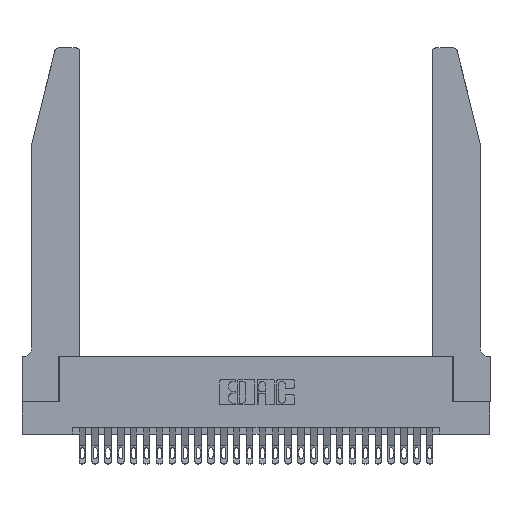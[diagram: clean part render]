
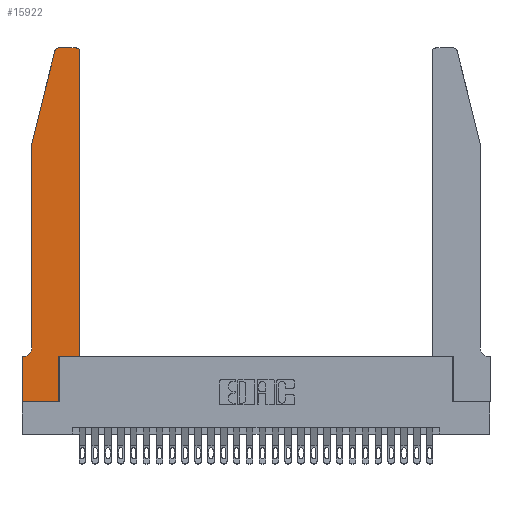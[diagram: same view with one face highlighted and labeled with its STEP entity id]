
A CAD part, top view. The second image highlights one B-rep face of the part: STEP entity #15922.
In plain terms, the highlighted planar face has unit normal (0, 0, 1).
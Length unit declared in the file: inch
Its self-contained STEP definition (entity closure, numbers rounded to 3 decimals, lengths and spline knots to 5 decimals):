
#129 = CARTESIAN_POINT ( 'NONE',  ( 0.2865, 0., 0.37 ) ) ;
#249 = CARTESIAN_POINT ( 'NONE',  ( 0.0755, 2., 0.37 ) ) ;
#687 = VERTEX_POINT ( 'NONE', #129 ) ;
#1228 = EDGE_LOOP ( 'NONE', ( #21166, #9160, #25264, #1572, #23077, #16402, #26009, #11171, #11777, #18417, #9724, #4285 ) ) ;
#1283 = AXIS2_PLACEMENT_3D ( 'NONE', #27763, #12015, #27660 ) ;
#1368 = AXIS2_PLACEMENT_3D ( 'NONE', #26612, #2082, #17727 ) ;
#1412 = DIRECTION ( 'NONE',  ( 1., 0., 0. ) ) ;
#1572 = ORIENTED_EDGE ( 'NONE', *, *, #11192, .T. ) ;
#2082 = DIRECTION ( 'NONE',  ( 0., 0., 1. ) ) ;
#2402 = CARTESIAN_POINT ( 'NONE',  ( 0.4205, 2.75, 0.37 ) ) ;
#2415 = DIRECTION ( 'NONE',  ( 0., -1., 0. ) ) ;
#2513 = AXIS2_PLACEMENT_3D ( 'NONE', #2610, #27211, #5008 ) ;
#2610 = CARTESIAN_POINT ( 'NONE',  ( 0.0055, 0.42, 0.37 ) ) ;
#2716 = LINE ( 'NONE', #18474, #7898 ) ;
#3113 = CARTESIAN_POINT ( 'NONE',  ( 0.2865, 0.35, 0.37 ) ) ;
#3643 = LINE ( 'NONE', #7606, #10619 ) ;
#3847 = VECTOR ( 'NONE', #25803, 39.37008 ) ;
#4285 = ORIENTED_EDGE ( 'NONE', *, *, #13616, .T. ) ;
#4448 = VECTOR ( 'NONE', #22983, 39.37008 ) ;
#4449 = CIRCLE ( 'NONE', #9726, 0.03 ) ;
#4637 = CARTESIAN_POINT ( 'NONE',  ( 0., 0., 0.37 ) ) ;
#5008 = DIRECTION ( 'NONE',  ( -1., 0., 0. ) ) ;
#5041 = CARTESIAN_POINT ( 'NONE',  ( 0.25487, 2.72718, 0.37 ) ) ;
#5281 = EDGE_CURVE ( 'NONE', #6188, #12179, #11892, .T. ) ;
#5611 = CIRCLE ( 'NONE', #1283, 0.03 ) ;
#5969 = CARTESIAN_POINT ( 'NONE',  ( 0., 0., 0.37 ) ) ;
#6003 = CARTESIAN_POINT ( 'NONE',  ( 0.4505, 2.72, 0.37 ) ) ;
#6188 = VERTEX_POINT ( 'NONE', #9576 ) ;
#6628 = VERTEX_POINT ( 'NONE', #5041 ) ;
#6860 = LINE ( 'NONE', #23150, #23339 ) ;
#6877 = EDGE_CURVE ( 'NONE', #20033, #6188, #6860, .T. ) ;
#7310 = CARTESIAN_POINT ( 'NONE',  ( 0.284, 2.75, 0.37 ) ) ;
#7357 = VECTOR ( 'NONE', #15889, 39.37008 ) ;
#7606 = CARTESIAN_POINT ( 'NONE',  ( 0.2605, 2.75, 0.37 ) ) ;
#7898 = VECTOR ( 'NONE', #9640, 39.37008 ) ;
#9097 = VERTEX_POINT ( 'NONE', #7310 ) ;
#9160 = ORIENTED_EDGE ( 'NONE', *, *, #10809, .T. ) ;
#9531 = CARTESIAN_POINT ( 'NONE',  ( 0.4505, 0.35, 0.37 ) ) ;
#9576 = CARTESIAN_POINT ( 'NONE',  ( 0., 0.35, 0.37 ) ) ;
#9640 = DIRECTION ( 'NONE',  ( -0.239, -0.971, 0. ) ) ;
#9724 = ORIENTED_EDGE ( 'NONE', *, *, #27611, .T. ) ;
#9726 = AXIS2_PLACEMENT_3D ( 'NONE', #25751, #28286, #1412 ) ;
#9915 = DIRECTION ( 'NONE',  ( 0., 1., 0. ) ) ;
#10619 = VECTOR ( 'NONE', #21056, 39.37008 ) ;
#10809 = EDGE_CURVE ( 'NONE', #9097, #6628, #5611, .T. ) ;
#11171 = ORIENTED_EDGE ( 'NONE', *, *, #19048, .T. ) ;
#11192 = EDGE_CURVE ( 'NONE', #23294, #23274, #15068, .T. ) ;
#11777 = ORIENTED_EDGE ( 'NONE', *, *, #17902, .T. ) ;
#11892 = LINE ( 'NONE', #4637, #16445 ) ;
#12015 = DIRECTION ( 'NONE',  ( 0., 0., 1. ) ) ;
#12179 = VERTEX_POINT ( 'NONE', #5969 ) ;
#13616 = EDGE_CURVE ( 'NONE', #23103, #15250, #4449, .T. ) ;
#13878 = CARTESIAN_POINT ( 'NONE',  ( 0., 0., 0.37 ) ) ;
#15068 = LINE ( 'NONE', #18067, #7357 ) ;
#15250 = VERTEX_POINT ( 'NONE', #2402 ) ;
#15889 = DIRECTION ( 'NONE',  ( 0., -1., 0. ) ) ;
#15922 = ADVANCED_FACE ( 'NONE', ( #28098 ), #24366, .T. ) ;
#16267 = DIRECTION ( 'NONE',  ( 1., 0., 0. ) ) ;
#16402 = ORIENTED_EDGE ( 'NONE', *, *, #6877, .T. ) ;
#16445 = VECTOR ( 'NONE', #2415, 39.37008 ) ;
#17727 = DIRECTION ( 'NONE',  ( 1., 0., 0. ) ) ;
#17902 = EDGE_CURVE ( 'NONE', #687, #27392, #23422, .T. ) ;
#18067 = CARTESIAN_POINT ( 'NONE',  ( 0.0755, 2., 0.37 ) ) ;
#18164 = CIRCLE ( 'NONE', #2513, 0.07 ) ;
#18413 = EDGE_CURVE ( 'NONE', #23274, #20033, #18164, .T. ) ;
#18417 = ORIENTED_EDGE ( 'NONE', *, *, #23461, .T. ) ;
#18474 = CARTESIAN_POINT ( 'NONE',  ( 0.0755, 2., 0.37 ) ) ;
#19048 = EDGE_CURVE ( 'NONE', #12179, #687, #28951, .T. ) ;
#19297 = LINE ( 'NONE', #23112, #26992 ) ;
#20033 = VERTEX_POINT ( 'NONE', #24849 ) ;
#20573 = LINE ( 'NONE', #23319, #25111 ) ;
#20588 = CARTESIAN_POINT ( 'NONE',  ( 0.0755, 0.42, 0.37 ) ) ;
#21056 = DIRECTION ( 'NONE',  ( -1., 0., 0. ) ) ;
#21166 = ORIENTED_EDGE ( 'NONE', *, *, #21408, .T. ) ;
#21287 = DIRECTION ( 'NONE',  ( -1., 0., 0. ) ) ;
#21408 = EDGE_CURVE ( 'NONE', #15250, #9097, #3643, .T. ) ;
#22268 = CARTESIAN_POINT ( 'NONE',  ( 0.2865, 0.35, 0.37 ) ) ;
#22873 = VERTEX_POINT ( 'NONE', #9531 ) ;
#22983 = DIRECTION ( 'NONE',  ( 1., 0., 0. ) ) ;
#23077 = ORIENTED_EDGE ( 'NONE', *, *, #18413, .T. ) ;
#23103 = VERTEX_POINT ( 'NONE', #6003 ) ;
#23112 = CARTESIAN_POINT ( 'NONE',  ( 0.4505, 0.35, 0.37 ) ) ;
#23150 = CARTESIAN_POINT ( 'NONE',  ( 0.0755, 0.35, 0.37 ) ) ;
#23274 = VERTEX_POINT ( 'NONE', #20588 ) ;
#23294 = VERTEX_POINT ( 'NONE', #249 ) ;
#23319 = CARTESIAN_POINT ( 'NONE',  ( 0.4505, 0.35, 0.37 ) ) ;
#23339 = VECTOR ( 'NONE', #21287, 39.37008 ) ;
#23422 = LINE ( 'NONE', #3113, #3847 ) ;
#23461 = EDGE_CURVE ( 'NONE', #27392, #22873, #19297, .T. ) ;
#24366 = PLANE ( 'NONE',  #1368 ) ;
#24849 = CARTESIAN_POINT ( 'NONE',  ( 0.0055, 0.35, 0.37 ) ) ;
#25111 = VECTOR ( 'NONE', #9915, 39.37008 ) ;
#25264 = ORIENTED_EDGE ( 'NONE', *, *, #28647, .T. ) ;
#25751 = CARTESIAN_POINT ( 'NONE',  ( 0.4205, 2.72, 0.37 ) ) ;
#25803 = DIRECTION ( 'NONE',  ( 0., 1., 0. ) ) ;
#26009 = ORIENTED_EDGE ( 'NONE', *, *, #5281, .T. ) ;
#26612 = CARTESIAN_POINT ( 'NONE',  ( 0., 0.35, 0.37 ) ) ;
#26992 = VECTOR ( 'NONE', #16267, 39.37008 ) ;
#27211 = DIRECTION ( 'NONE',  ( 0., 0., -1. ) ) ;
#27392 = VERTEX_POINT ( 'NONE', #22268 ) ;
#27611 = EDGE_CURVE ( 'NONE', #22873, #23103, #20573, .T. ) ;
#27660 = DIRECTION ( 'NONE',  ( 1., 0., 0. ) ) ;
#27763 = CARTESIAN_POINT ( 'NONE',  ( 0.284, 2.72, 0.37 ) ) ;
#28098 = FACE_OUTER_BOUND ( 'NONE', #1228, .T. ) ;
#28286 = DIRECTION ( 'NONE',  ( 0., 0., 1. ) ) ;
#28647 = EDGE_CURVE ( 'NONE', #6628, #23294, #2716, .T. ) ;
#28951 = LINE ( 'NONE', #13878, #4448 ) ;
